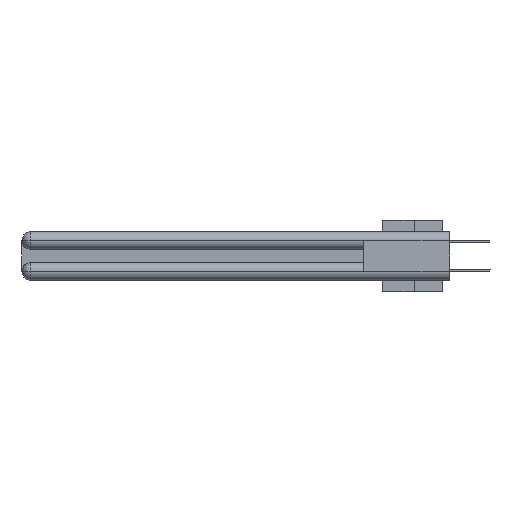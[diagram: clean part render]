
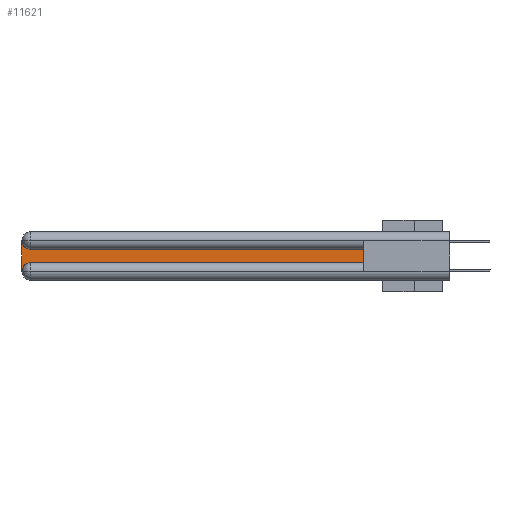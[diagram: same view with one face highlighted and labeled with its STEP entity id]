
A CAD part, left-side view. The second image highlights one B-rep face of the part: STEP entity #11621.
In plain terms, the highlighted planar face has unit normal (-1, 0, 0).
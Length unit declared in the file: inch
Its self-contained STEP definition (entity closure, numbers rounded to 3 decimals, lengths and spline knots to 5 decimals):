
#1147 = ORIENTED_EDGE ( 'NONE', *, *, #32660, .T. ) ;
#2013 = DIRECTION ( 'NONE',  ( 0., 1., 0. ) ) ;
#2303 = DIRECTION ( 'NONE',  ( 1., 0., 0. ) ) ;
#2324 = LINE ( 'NONE', #31236, #5036 ) ;
#2811 = ORIENTED_EDGE ( 'NONE', *, *, #12208, .T. ) ;
#2997 = AXIS2_PLACEMENT_3D ( 'NONE', #17688, #26655, #23855 ) ;
#3092 = EDGE_LOOP ( 'NONE', ( #2811, #33349, #33041, #30923, #5864, #1147 ) ) ;
#4613 = VERTEX_POINT ( 'NONE', #35219 ) ;
#4686 = LINE ( 'NONE', #16142, #33780 ) ;
#5036 = VECTOR ( 'NONE', #21918, 39.37008 ) ;
#5116 = LINE ( 'NONE', #10852, #7837 ) ;
#5599 = CIRCLE ( 'NONE', #7757, 0.06 ) ;
#5864 = ORIENTED_EDGE ( 'NONE', *, *, #31803, .T. ) ;
#7150 = DIRECTION ( 'NONE',  ( 0., 0., -1. ) ) ;
#7757 = AXIS2_PLACEMENT_3D ( 'NONE', #22789, #2303, #16753 ) ;
#7824 = VECTOR ( 'NONE', #7150, 39.37008 ) ;
#7837 = VECTOR ( 'NONE', #2013, 39.37008 ) ;
#9881 = VERTEX_POINT ( 'NONE', #11689 ) ;
#10209 = CARTESIAN_POINT ( 'NONE',  ( 0.075, 3., -0.2175 ) ) ;
#10852 = CARTESIAN_POINT ( 'NONE',  ( 0.075, 0.6, -0.1225 ) ) ;
#11420 = AXIS2_PLACEMENT_3D ( 'NONE', #27331, #27477, #27207 ) ;
#11621 = ADVANCED_FACE ( 'NONE', ( #16045 ), #15911, .F. ) ;
#11689 = CARTESIAN_POINT ( 'NONE',  ( 0.075, 2.94, -0.2175 ) ) ;
#12208 = EDGE_CURVE ( 'NONE', #29426, #27179, #5116, .T. ) ;
#13740 = EDGE_CURVE ( 'NONE', #27179, #31552, #36890, .T. ) ;
#14104 = CARTESIAN_POINT ( 'NONE',  ( 0.075, 0.6, -0.1225 ) ) ;
#14312 = CARTESIAN_POINT ( 'NONE',  ( 0.075, 3., -0.0625 ) ) ;
#14636 = LINE ( 'NONE', #10209, #7824 ) ;
#15911 = PLANE ( 'NONE',  #11420 ) ;
#16045 = FACE_OUTER_BOUND ( 'NONE', #3092, .T. ) ;
#16142 = CARTESIAN_POINT ( 'NONE',  ( 0.075, 0.6, -0.2175 ) ) ;
#16753 = DIRECTION ( 'NONE',  ( 0., 0., -1. ) ) ;
#17036 = CARTESIAN_POINT ( 'NONE',  ( 0.075, 3., -0.2775 ) ) ;
#17074 = VERTEX_POINT ( 'NONE', #17036 ) ;
#17688 = CARTESIAN_POINT ( 'NONE',  ( 0.075, 2.94, -0.0625 ) ) ;
#20760 = EDGE_CURVE ( 'NONE', #17074, #9881, #5599, .T. ) ;
#21268 = EDGE_CURVE ( 'NONE', #31552, #17074, #14636, .T. ) ;
#21918 = DIRECTION ( 'NONE',  ( 0., 0., 1. ) ) ;
#22789 = CARTESIAN_POINT ( 'NONE',  ( 0.075, 2.94, -0.2775 ) ) ;
#23855 = DIRECTION ( 'NONE',  ( 0., 0., -1. ) ) ;
#25134 = DIRECTION ( 'NONE',  ( 0., -1., 0. ) ) ;
#26655 = DIRECTION ( 'NONE',  ( 1., 0., 0. ) ) ;
#27179 = VERTEX_POINT ( 'NONE', #37615 ) ;
#27207 = DIRECTION ( 'NONE',  ( 0., 0., -1. ) ) ;
#27331 = CARTESIAN_POINT ( 'NONE',  ( 0.075, 3., -0.1225 ) ) ;
#27477 = DIRECTION ( 'NONE',  ( 1., 0., 0. ) ) ;
#29426 = VERTEX_POINT ( 'NONE', #14104 ) ;
#30923 = ORIENTED_EDGE ( 'NONE', *, *, #20760, .T. ) ;
#31236 = CARTESIAN_POINT ( 'NONE',  ( 0.075, 0.6, -0.2175 ) ) ;
#31552 = VERTEX_POINT ( 'NONE', #14312 ) ;
#31803 = EDGE_CURVE ( 'NONE', #9881, #4613, #4686, .T. ) ;
#32660 = EDGE_CURVE ( 'NONE', #4613, #29426, #2324, .T. ) ;
#33041 = ORIENTED_EDGE ( 'NONE', *, *, #21268, .T. ) ;
#33349 = ORIENTED_EDGE ( 'NONE', *, *, #13740, .T. ) ;
#33780 = VECTOR ( 'NONE', #25134, 39.37008 ) ;
#35219 = CARTESIAN_POINT ( 'NONE',  ( 0.075, 0.6, -0.2175 ) ) ;
#36890 = CIRCLE ( 'NONE', #2997, 0.06 ) ;
#37615 = CARTESIAN_POINT ( 'NONE',  ( 0.075, 2.94, -0.1225 ) ) ;
